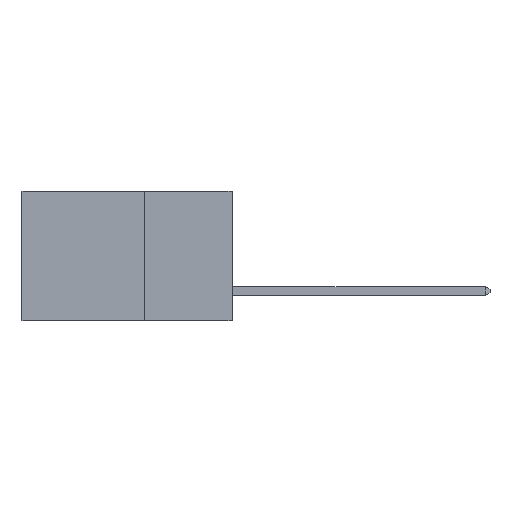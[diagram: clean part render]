
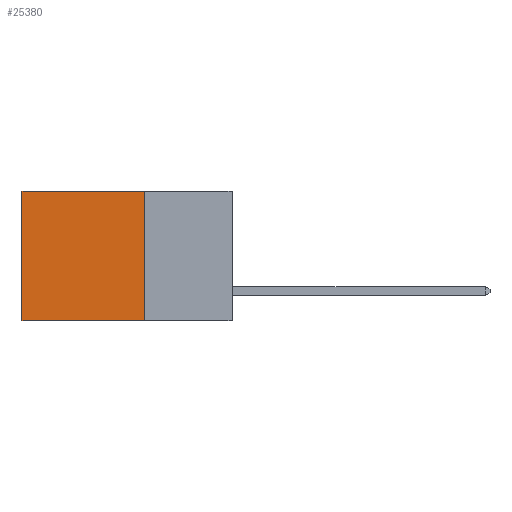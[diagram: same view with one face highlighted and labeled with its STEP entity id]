
A CAD part, left-side view. The second image highlights one B-rep face of the part: STEP entity #25380.
In plain terms, the highlighted planar face has unit normal (-1, 0, 0).
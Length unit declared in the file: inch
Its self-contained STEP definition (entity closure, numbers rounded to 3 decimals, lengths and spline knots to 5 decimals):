
#38 = VERTEX_POINT ( 'NONE', #21061 ) ;
#82 = VECTOR ( 'NONE', #22764, 39.37008 ) ;
#982 = LINE ( 'NONE', #28050, #12902 ) ;
#1320 = CARTESIAN_POINT ( 'NONE',  ( 0.2875, 0.6, 0. ) ) ;
#1938 = EDGE_CURVE ( 'NONE', #23435, #38, #4228, .T. ) ;
#3260 = AXIS2_PLACEMENT_3D ( 'NONE', #27831, #18366, #4118 ) ;
#3739 = CARTESIAN_POINT ( 'NONE',  ( 0.2875, 0.25, 0. ) ) ;
#4118 = DIRECTION ( 'NONE',  ( 0., 0., -1. ) ) ;
#4228 = LINE ( 'NONE', #9526, #28774 ) ;
#7817 = ORIENTED_EDGE ( 'NONE', *, *, #1938, .F. ) ;
#9526 = CARTESIAN_POINT ( 'NONE',  ( 0.2875, 0.25, 0. ) ) ;
#9877 = FACE_OUTER_BOUND ( 'NONE', #20465, .T. ) ;
#12902 = VECTOR ( 'NONE', #23383, 39.37008 ) ;
#14454 = EDGE_CURVE ( 'NONE', #23435, #25245, #25375, .T. ) ;
#15990 = PLANE ( 'NONE',  #3260 ) ;
#16363 = VERTEX_POINT ( 'NONE', #30112 ) ;
#18338 = EDGE_CURVE ( 'NONE', #25245, #16363, #982, .T. ) ;
#18366 = DIRECTION ( 'NONE',  ( 1., 0., 0. ) ) ;
#19069 = DIRECTION ( 'NONE',  ( 0., 0., -1. ) ) ;
#20465 = EDGE_LOOP ( 'NONE', ( #29844, #24386, #7817, #21686 ) ) ;
#20661 = CARTESIAN_POINT ( 'NONE',  ( 0.2875, 0.25, 0. ) ) ;
#21061 = CARTESIAN_POINT ( 'NONE',  ( 0.2875, 0.25, -0.37 ) ) ;
#21686 = ORIENTED_EDGE ( 'NONE', *, *, #14454, .T. ) ;
#22764 = DIRECTION ( 'NONE',  ( 0., 1., 0. ) ) ;
#23383 = DIRECTION ( 'NONE',  ( 0., 0., -1. ) ) ;
#23435 = VERTEX_POINT ( 'NONE', #20661 ) ;
#24386 = ORIENTED_EDGE ( 'NONE', *, *, #25646, .F. ) ;
#25245 = VERTEX_POINT ( 'NONE', #1320 ) ;
#25375 = LINE ( 'NONE', #3739, #82 ) ;
#25380 = ADVANCED_FACE ( 'NONE', ( #9877 ), #15990, .F. ) ;
#25646 = EDGE_CURVE ( 'NONE', #38, #16363, #27692, .T. ) ;
#26781 = DIRECTION ( 'NONE',  ( 0., 1., 0. ) ) ;
#27692 = LINE ( 'NONE', #29063, #28444 ) ;
#27831 = CARTESIAN_POINT ( 'NONE',  ( 0.2875, 0.25, 0. ) ) ;
#28050 = CARTESIAN_POINT ( 'NONE',  ( 0.2875, 0.6, 0. ) ) ;
#28444 = VECTOR ( 'NONE', #26781, 39.37008 ) ;
#28774 = VECTOR ( 'NONE', #19069, 39.37008 ) ;
#29063 = CARTESIAN_POINT ( 'NONE',  ( 0.2875, 0.25, -0.37 ) ) ;
#29844 = ORIENTED_EDGE ( 'NONE', *, *, #18338, .T. ) ;
#30112 = CARTESIAN_POINT ( 'NONE',  ( 0.2875, 0.6, -0.37 ) ) ;
